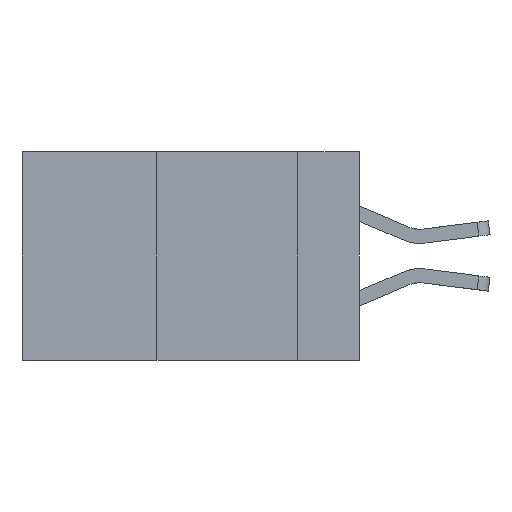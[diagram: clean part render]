
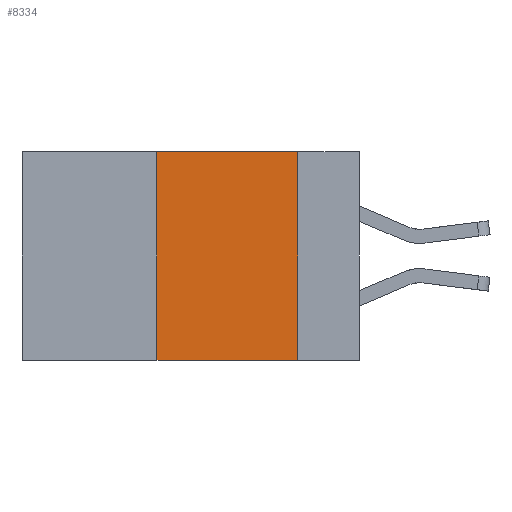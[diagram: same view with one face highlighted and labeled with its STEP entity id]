
A CAD part, left-side view. The second image highlights one B-rep face of the part: STEP entity #8334.
In plain terms, the highlighted planar face has unit normal (-1, 0, 0).
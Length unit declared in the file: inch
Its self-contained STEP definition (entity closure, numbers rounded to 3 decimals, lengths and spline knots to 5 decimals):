
#656 = LINE ( 'NONE', #14236, #12797 ) ;
#1256 = CARTESIAN_POINT ( 'NONE',  ( 0., 0.11, 0. ) ) ;
#1358 = DIRECTION ( 'NONE',  ( 0., 0., 1. ) ) ;
#1448 = CARTESIAN_POINT ( 'NONE',  ( 0., 0.36, 0. ) ) ;
#1598 = EDGE_CURVE ( 'NONE', #2866, #11486, #656, .T. ) ;
#2330 = ORIENTED_EDGE ( 'NONE', *, *, #9448, .T. ) ;
#2866 = VERTEX_POINT ( 'NONE', #1256 ) ;
#3178 = LINE ( 'NONE', #1448, #9010 ) ;
#3466 = ORIENTED_EDGE ( 'NONE', *, *, #6203, .F. ) ;
#3514 = VECTOR ( 'NONE', #12021, 39.37008 ) ;
#4453 = FACE_OUTER_BOUND ( 'NONE', #7564, .T. ) ;
#5417 = CARTESIAN_POINT ( 'NONE',  ( 0., 0.11, -0.37 ) ) ;
#5472 = ORIENTED_EDGE ( 'NONE', *, *, #14174, .F. ) ;
#5697 = AXIS2_PLACEMENT_3D ( 'NONE', #13299, #14461, #7455 ) ;
#6203 = EDGE_CURVE ( 'NONE', #11317, #11425, #3178, .T. ) ;
#6298 = CARTESIAN_POINT ( 'NONE',  ( 0., 0.36, -0.37 ) ) ;
#6402 = ORIENTED_EDGE ( 'NONE', *, *, #1598, .F. ) ;
#7455 = DIRECTION ( 'NONE',  ( 0., 0., -1. ) ) ;
#7564 = EDGE_LOOP ( 'NONE', ( #6402, #5472, #3466, #2330 ) ) ;
#7718 = LINE ( 'NONE', #14347, #3514 ) ;
#8334 = ADVANCED_FACE ( 'NONE', ( #4453 ), #12095, .F. ) ;
#8763 = LINE ( 'NONE', #10002, #14618 ) ;
#9010 = VECTOR ( 'NONE', #1358, 39.37008 ) ;
#9448 = EDGE_CURVE ( 'NONE', #11317, #11486, #7718, .T. ) ;
#10002 = CARTESIAN_POINT ( 'NONE',  ( 0., 0.6, 0. ) ) ;
#11317 = VERTEX_POINT ( 'NONE', #6298 ) ;
#11425 = VERTEX_POINT ( 'NONE', #14645 ) ;
#11486 = VERTEX_POINT ( 'NONE', #5417 ) ;
#12021 = DIRECTION ( 'NONE',  ( 0., -1., 0. ) ) ;
#12095 = PLANE ( 'NONE',  #5697 ) ;
#12797 = VECTOR ( 'NONE', #14289, 39.37008 ) ;
#13299 = CARTESIAN_POINT ( 'NONE',  ( 0., 0.6, 0. ) ) ;
#14174 = EDGE_CURVE ( 'NONE', #11425, #2866, #8763, .T. ) ;
#14236 = CARTESIAN_POINT ( 'NONE',  ( 0., 0.11, 0. ) ) ;
#14289 = DIRECTION ( 'NONE',  ( 0., 0., -1. ) ) ;
#14347 = CARTESIAN_POINT ( 'NONE',  ( 0., 0.6, -0.37 ) ) ;
#14461 = DIRECTION ( 'NONE',  ( 1., 0., 0. ) ) ;
#14618 = VECTOR ( 'NONE', #14749, 39.37008 ) ;
#14645 = CARTESIAN_POINT ( 'NONE',  ( 0., 0.36, 0. ) ) ;
#14749 = DIRECTION ( 'NONE',  ( 0., -1., 0. ) ) ;
